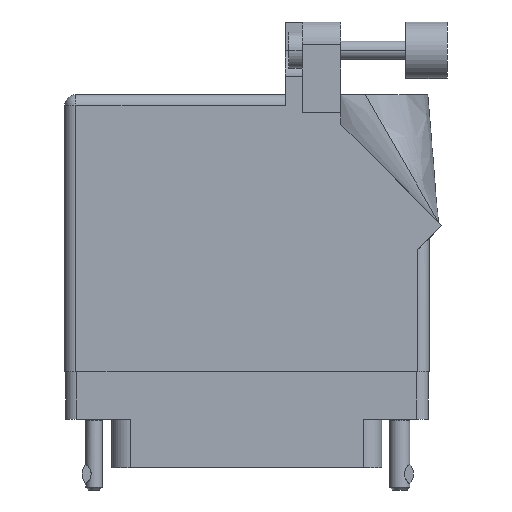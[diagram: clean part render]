
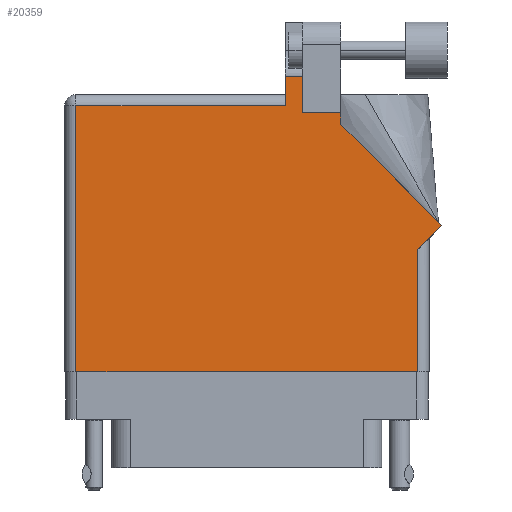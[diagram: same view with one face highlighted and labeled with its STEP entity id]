
A CAD part, front view. The second image highlights one B-rep face of the part: STEP entity #20359.
In plain terms, the highlighted face is planar.
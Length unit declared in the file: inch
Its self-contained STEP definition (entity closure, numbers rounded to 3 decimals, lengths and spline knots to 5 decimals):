
#715 = EDGE_CURVE ( 'NONE', #4632, #48105, #5731, .T. ) ;
#738 = VERTEX_POINT ( 'NONE', #16315 ) ;
#2157 = EDGE_CURVE ( 'NONE', #34108, #13624, #45434, .T. ) ;
#2235 = EDGE_LOOP ( 'NONE', ( #22994, #7078, #16921, #5538, #38474, #16710, #11420, #32761, #18683, #27757, #24867 ) ) ;
#2741 = EDGE_CURVE ( 'NONE', #41540, #23536, #48288, .T. ) ;
#3099 = LINE ( 'NONE', #37978, #17155 ) ;
#3155 = PLANE ( 'NONE',  #3944 ) ;
#3283 = VECTOR ( 'NONE', #41486, 39.37008 ) ;
#3824 = LINE ( 'NONE', #8055, #26028 ) ;
#3918 = CARTESIAN_POINT ( 'NONE',  ( 0., 0., 0. ) ) ;
#3944 = AXIS2_PLACEMENT_3D ( 'NONE', #10672, #15097, #26548 ) ;
#4368 = VERTEX_POINT ( 'NONE', #13212 ) ;
#4632 = VERTEX_POINT ( 'NONE', #14532 ) ;
#5416 = CARTESIAN_POINT ( 'NONE',  ( 0.062, 0., 0. ) ) ;
#5538 = ORIENTED_EDGE ( 'NONE', *, *, #2741, .T. ) ;
#5681 = VERTEX_POINT ( 'NONE', #43180 ) ;
#5702 = CARTESIAN_POINT ( 'NONE',  ( 1.311, 1.43, 0. ) ) ;
#5731 = LINE ( 'NONE', #42447, #44318 ) ;
#6563 = CARTESIAN_POINT ( 'NONE',  ( 1.948, 0., 0. ) ) ;
#6678 = LINE ( 'NONE', #25372, #31288 ) ;
#6923 = VECTOR ( 'NONE', #8851, 39.37008 ) ;
#7078 = ORIENTED_EDGE ( 'NONE', *, *, #715, .T. ) ;
#8055 = CARTESIAN_POINT ( 'NONE',  ( 1.217, 1.53, 0. ) ) ;
#8851 = DIRECTION ( 'NONE',  ( 0., -1., 0. ) ) ;
#9782 = VECTOR ( 'NONE', #48497, 39.37008 ) ;
#10672 = CARTESIAN_POINT ( 'NONE',  ( 0., 1.53, 0. ) ) ;
#11273 = EDGE_CURVE ( 'NONE', #738, #4632, #41892, .T. ) ;
#11420 = ORIENTED_EDGE ( 'NONE', *, *, #26252, .T. ) ;
#11487 = EDGE_CURVE ( 'NONE', #4368, #5681, #16145, .T. ) ;
#12310 = EDGE_CURVE ( 'NONE', #48105, #41540, #3824, .T. ) ;
#12550 = EDGE_CURVE ( 'NONE', #19400, #4368, #6678, .T. ) ;
#12671 = LINE ( 'NONE', #44396, #9782 ) ;
#13212 = CARTESIAN_POINT ( 'NONE',  ( 1.524, 1.36442, 0. ) ) ;
#13624 = VERTEX_POINT ( 'NONE', #6563 ) ;
#14532 = CARTESIAN_POINT ( 'NONE',  ( 1.311, 1.6315, 0. ) ) ;
#15097 = DIRECTION ( 'NONE',  ( 0., 0., -1. ) ) ;
#16145 = LINE ( 'NONE', #40658, #47717 ) ;
#16315 = CARTESIAN_POINT ( 'NONE',  ( 1.311, 1.43, 0. ) ) ;
#16710 = ORIENTED_EDGE ( 'NONE', *, *, #2157, .T. ) ;
#16921 = ORIENTED_EDGE ( 'NONE', *, *, #12310, .T. ) ;
#17155 = VECTOR ( 'NONE', #41848, 39.37008 ) ;
#18568 = CARTESIAN_POINT ( 'NONE',  ( 2.01, 0.737, 0. ) ) ;
#18683 = ORIENTED_EDGE ( 'NONE', *, *, #12550, .T. ) ;
#18958 = FACE_OUTER_BOUND ( 'NONE', #2235, .T. ) ;
#19359 = DIRECTION ( 'NONE',  ( 0., -1., 0. ) ) ;
#19400 = VERTEX_POINT ( 'NONE', #24503 ) ;
#20359 = ADVANCED_FACE ( 'NONE', ( #18958 ), #3155, .F. ) ;
#20380 = CARTESIAN_POINT ( 'NONE',  ( 0.062, 0., 0. ) ) ;
#21702 = LINE ( 'NONE', #18568, #30517 ) ;
#22636 = CARTESIAN_POINT ( 'NONE',  ( 1.948, 0.675, 0. ) ) ;
#22994 = ORIENTED_EDGE ( 'NONE', *, *, #11273, .T. ) ;
#23103 = EDGE_CURVE ( 'NONE', #43447, #19400, #21702, .T. ) ;
#23536 = VERTEX_POINT ( 'NONE', #36345 ) ;
#23837 = DIRECTION ( 'NONE',  ( -1., 0., 0. ) ) ;
#24503 = CARTESIAN_POINT ( 'NONE',  ( 2.08071, 0.80771, 0. ) ) ;
#24867 = ORIENTED_EDGE ( 'NONE', *, *, #31315, .T. ) ;
#25205 = DIRECTION ( 'NONE',  ( -0.707, 0.707, 0. ) ) ;
#25372 = CARTESIAN_POINT ( 'NONE',  ( 2.08071, 0.80771, 0. ) ) ;
#25540 = VECTOR ( 'NONE', #27960, 39.37008 ) ;
#25570 = DIRECTION ( 'NONE',  ( 0.707, 0.707, 0. ) ) ;
#26028 = VECTOR ( 'NONE', #19359, 39.37008 ) ;
#26252 = EDGE_CURVE ( 'NONE', #13624, #43447, #3099, .T. ) ;
#26548 = DIRECTION ( 'NONE',  ( -1., 0., 0. ) ) ;
#27757 = ORIENTED_EDGE ( 'NONE', *, *, #11487, .T. ) ;
#27960 = DIRECTION ( 'NONE',  ( 0., 1., 0. ) ) ;
#30276 = EDGE_CURVE ( 'NONE', #23536, #34108, #33282, .T. ) ;
#30517 = VECTOR ( 'NONE', #25570, 39.37008 ) ;
#31288 = VECTOR ( 'NONE', #25205, 39.37008 ) ;
#31315 = EDGE_CURVE ( 'NONE', #5681, #738, #12671, .T. ) ;
#32761 = ORIENTED_EDGE ( 'NONE', *, *, #23103, .T. ) ;
#33282 = LINE ( 'NONE', #5416, #6923 ) ;
#34108 = VERTEX_POINT ( 'NONE', #20380 ) ;
#36345 = CARTESIAN_POINT ( 'NONE',  ( 0.062, 1.468, 0. ) ) ;
#37085 = DIRECTION ( 'NONE',  ( 0., 1., 0. ) ) ;
#37978 = CARTESIAN_POINT ( 'NONE',  ( 1.948, 0.737, 0. ) ) ;
#38361 = VECTOR ( 'NONE', #42407, 39.37008 ) ;
#38474 = ORIENTED_EDGE ( 'NONE', *, *, #30276, .T. ) ;
#38934 = CARTESIAN_POINT ( 'NONE',  ( 1.217, 1.468, 0. ) ) ;
#39194 = CARTESIAN_POINT ( 'NONE',  ( 1.217, 1.6315, 0. ) ) ;
#40658 = CARTESIAN_POINT ( 'NONE',  ( 1.524, 1.36442, 0. ) ) ;
#41486 = DIRECTION ( 'NONE',  ( 1., 0., 0. ) ) ;
#41540 = VERTEX_POINT ( 'NONE', #38934 ) ;
#41848 = DIRECTION ( 'NONE',  ( 0., 1., 0. ) ) ;
#41892 = LINE ( 'NONE', #5702, #25540 ) ;
#42407 = DIRECTION ( 'NONE',  ( -1., 0., 0. ) ) ;
#42447 = CARTESIAN_POINT ( 'NONE',  ( 1.64177, 1.6315, 0. ) ) ;
#43180 = CARTESIAN_POINT ( 'NONE',  ( 1.524, 1.43, 0. ) ) ;
#43447 = VERTEX_POINT ( 'NONE', #22636 ) ;
#44318 = VECTOR ( 'NONE', #23837, 39.37008 ) ;
#44396 = CARTESIAN_POINT ( 'NONE',  ( 1.524, 1.43, 0. ) ) ;
#45434 = LINE ( 'NONE', #3918, #3283 ) ;
#46192 = CARTESIAN_POINT ( 'NONE',  ( 0., 1.468, 0. ) ) ;
#47717 = VECTOR ( 'NONE', #37085, 39.37008 ) ;
#48105 = VERTEX_POINT ( 'NONE', #39194 ) ;
#48288 = LINE ( 'NONE', #46192, #38361 ) ;
#48497 = DIRECTION ( 'NONE',  ( -1., 0., 0. ) ) ;
